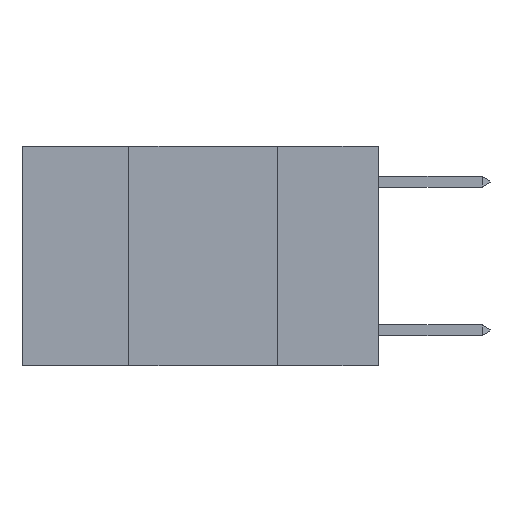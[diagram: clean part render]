
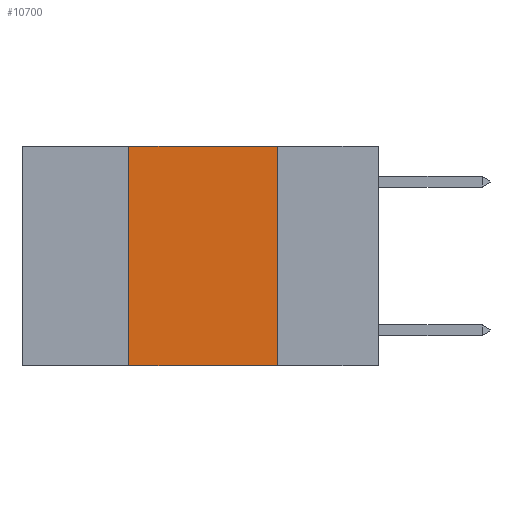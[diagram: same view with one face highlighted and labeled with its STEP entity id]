
A CAD part, left-side view. The second image highlights one B-rep face of the part: STEP entity #10700.
In plain terms, the highlighted planar face has unit normal (-1, 0, 0).
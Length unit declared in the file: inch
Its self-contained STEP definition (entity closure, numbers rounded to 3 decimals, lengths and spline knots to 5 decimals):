
#184 = ORIENTED_EDGE ( 'NONE', *, *, #10543, .F. ) ;
#317 = EDGE_LOOP ( 'NONE', ( #184, #4906, #10106, #3065 ) ) ;
#495 = DIRECTION ( 'NONE',  ( 0., 0., 1. ) ) ;
#727 = VERTEX_POINT ( 'NONE', #10792 ) ;
#1524 = LINE ( 'NONE', #10442, #1763 ) ;
#1763 = VECTOR ( 'NONE', #6920, 39.37008 ) ;
#1770 = EDGE_CURVE ( 'NONE', #7937, #2037, #1524, .T. ) ;
#2037 = VERTEX_POINT ( 'NONE', #6571 ) ;
#2211 = VECTOR ( 'NONE', #10508, 39.37008 ) ;
#2265 = CARTESIAN_POINT ( 'NONE',  ( 0., 0.42, 0. ) ) ;
#2387 = CARTESIAN_POINT ( 'NONE',  ( 0., 0.42, 0. ) ) ;
#3065 = ORIENTED_EDGE ( 'NONE', *, *, #7597, .T. ) ;
#3758 = PLANE ( 'NONE',  #11140 ) ;
#4672 = FACE_OUTER_BOUND ( 'NONE', #317, .T. ) ;
#4736 = CARTESIAN_POINT ( 'NONE',  ( 0., 0.6, 0. ) ) ;
#4906 = ORIENTED_EDGE ( 'NONE', *, *, #1770, .F. ) ;
#5014 = VECTOR ( 'NONE', #495, 39.37008 ) ;
#5257 = LINE ( 'NONE', #6931, #2211 ) ;
#5656 = DIRECTION ( 'NONE',  ( 0., 0., -1. ) ) ;
#6210 = CARTESIAN_POINT ( 'NONE',  ( 0., 0.6, -0.37 ) ) ;
#6571 = CARTESIAN_POINT ( 'NONE',  ( 0., 0.17, 0. ) ) ;
#6920 = DIRECTION ( 'NONE',  ( 0., -1., 0. ) ) ;
#6931 = CARTESIAN_POINT ( 'NONE',  ( 0., 0.17, 0. ) ) ;
#7224 = DIRECTION ( 'NONE',  ( 1., 0., 0. ) ) ;
#7597 = EDGE_CURVE ( 'NONE', #11037, #727, #7921, .T. ) ;
#7921 = LINE ( 'NONE', #6210, #10791 ) ;
#7937 = VERTEX_POINT ( 'NONE', #2387 ) ;
#8405 = EDGE_CURVE ( 'NONE', #11037, #7937, #8470, .T. ) ;
#8470 = LINE ( 'NONE', #2265, #5014 ) ;
#8781 = DIRECTION ( 'NONE',  ( 0., -1., 0. ) ) ;
#9150 = CARTESIAN_POINT ( 'NONE',  ( 0., 0.42, -0.37 ) ) ;
#10106 = ORIENTED_EDGE ( 'NONE', *, *, #8405, .F. ) ;
#10442 = CARTESIAN_POINT ( 'NONE',  ( 0., 0.6, 0. ) ) ;
#10508 = DIRECTION ( 'NONE',  ( 0., 0., -1. ) ) ;
#10543 = EDGE_CURVE ( 'NONE', #2037, #727, #5257, .T. ) ;
#10700 = ADVANCED_FACE ( 'NONE', ( #4672 ), #3758, .F. ) ;
#10791 = VECTOR ( 'NONE', #8781, 39.37008 ) ;
#10792 = CARTESIAN_POINT ( 'NONE',  ( 0., 0.17, -0.37 ) ) ;
#11037 = VERTEX_POINT ( 'NONE', #9150 ) ;
#11140 = AXIS2_PLACEMENT_3D ( 'NONE', #4736, #7224, #5656 ) ;
